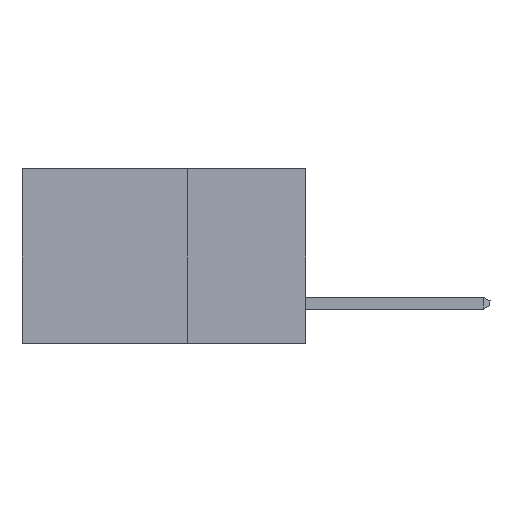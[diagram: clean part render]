
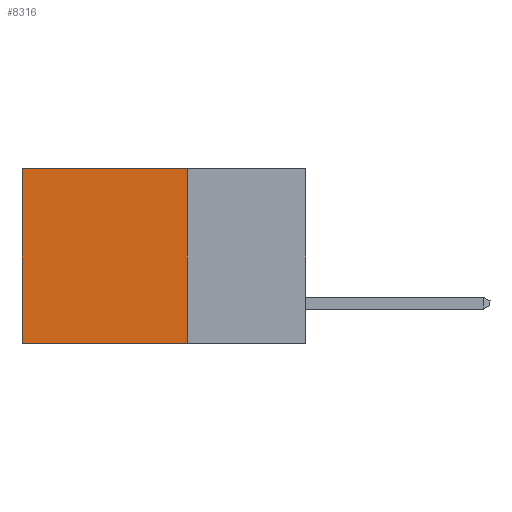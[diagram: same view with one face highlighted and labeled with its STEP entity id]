
A CAD part, left-side view. The second image highlights one B-rep face of the part: STEP entity #8316.
In plain terms, the highlighted planar face has unit normal (-1, 0, 0).
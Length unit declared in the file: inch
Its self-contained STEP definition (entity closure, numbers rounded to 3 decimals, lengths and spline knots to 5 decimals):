
#656 = ORIENTED_EDGE ( 'NONE', *, *, #8836, .F. ) ;
#908 = ORIENTED_EDGE ( 'NONE', *, *, #15587, .F. ) ;
#1422 = CARTESIAN_POINT ( 'NONE',  ( 0.2615, 0.25, 0. ) ) ;
#2085 = EDGE_CURVE ( 'NONE', #13755, #12948, #6988, .T. ) ;
#2752 = FACE_OUTER_BOUND ( 'NONE', #9894, .T. ) ;
#2786 = LINE ( 'NONE', #14175, #6461 ) ;
#4050 = EDGE_CURVE ( 'NONE', #12948, #10216, #15293, .T. ) ;
#4155 = VECTOR ( 'NONE', #5415, 39.37008 ) ;
#4236 = PLANE ( 'NONE',  #16979 ) ;
#4652 = VERTEX_POINT ( 'NONE', #14647 ) ;
#5228 = CARTESIAN_POINT ( 'NONE',  ( 0.2615, 0.25, 0. ) ) ;
#5415 = DIRECTION ( 'NONE',  ( 0., 0., -1. ) ) ;
#5668 = DIRECTION ( 'NONE',  ( 0., 0., -1. ) ) ;
#6461 = VECTOR ( 'NONE', #9979, 39.37008 ) ;
#6988 = LINE ( 'NONE', #5228, #12148 ) ;
#7468 = LINE ( 'NONE', #11570, #15367 ) ;
#8316 = ADVANCED_FACE ( 'NONE', ( #2752 ), #4236, .F. ) ;
#8769 = DIRECTION ( 'NONE',  ( 0., 0., -1. ) ) ;
#8836 = EDGE_CURVE ( 'NONE', #4652, #10216, #2786, .T. ) ;
#9029 = CARTESIAN_POINT ( 'NONE',  ( 0.2615, 0.6, 0. ) ) ;
#9865 = CARTESIAN_POINT ( 'NONE',  ( 0.2615, 0.25, -0.37 ) ) ;
#9894 = EDGE_LOOP ( 'NONE', ( #15164, #656, #908, #12707 ) ) ;
#9979 = DIRECTION ( 'NONE',  ( 0., 1., 0. ) ) ;
#10216 = VERTEX_POINT ( 'NONE', #11129 ) ;
#11129 = CARTESIAN_POINT ( 'NONE',  ( 0.2615, 0.6, -0.37 ) ) ;
#11570 = CARTESIAN_POINT ( 'NONE',  ( 0.2615, 0.25, -0.37 ) ) ;
#12148 = VECTOR ( 'NONE', #16611, 39.37008 ) ;
#12632 = DIRECTION ( 'NONE',  ( 1., 0., 0. ) ) ;
#12707 = ORIENTED_EDGE ( 'NONE', *, *, #2085, .T. ) ;
#12948 = VERTEX_POINT ( 'NONE', #9029 ) ;
#13755 = VERTEX_POINT ( 'NONE', #1422 ) ;
#13882 = CARTESIAN_POINT ( 'NONE',  ( 0.2615, 0.6, -0.37 ) ) ;
#14175 = CARTESIAN_POINT ( 'NONE',  ( 0.2615, 0.25, -0.37 ) ) ;
#14647 = CARTESIAN_POINT ( 'NONE',  ( 0.2615, 0.25, -0.37 ) ) ;
#15164 = ORIENTED_EDGE ( 'NONE', *, *, #4050, .T. ) ;
#15293 = LINE ( 'NONE', #13882, #4155 ) ;
#15367 = VECTOR ( 'NONE', #8769, 39.37008 ) ;
#15587 = EDGE_CURVE ( 'NONE', #13755, #4652, #7468, .T. ) ;
#16611 = DIRECTION ( 'NONE',  ( 0., 1., 0. ) ) ;
#16979 = AXIS2_PLACEMENT_3D ( 'NONE', #9865, #12632, #5668 ) ;
